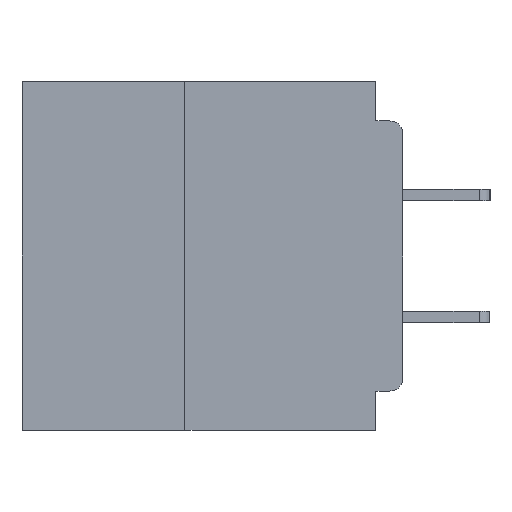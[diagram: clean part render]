
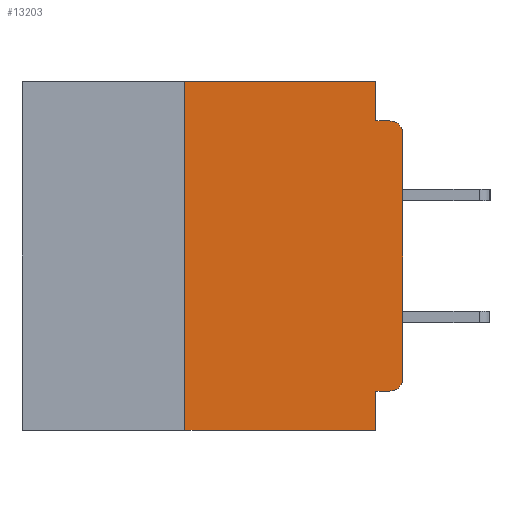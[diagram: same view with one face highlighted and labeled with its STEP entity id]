
A CAD part, left-side view. The second image highlights one B-rep face of the part: STEP entity #13203.
In plain terms, the highlighted planar face has unit normal (-1, 0, 0).
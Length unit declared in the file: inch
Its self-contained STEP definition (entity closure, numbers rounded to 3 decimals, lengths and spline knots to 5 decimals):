
#401 = VERTEX_POINT ( 'NONE', #18178 ) ;
#809 = ORIENTED_EDGE ( 'NONE', *, *, #40413, .F. ) ;
#1559 = EDGE_CURVE ( 'NONE', #32634, #18554, #17496, .T. ) ;
#2221 = CARTESIAN_POINT ( 'NONE',  ( 0., 0.25, 0. ) ) ;
#2320 = EDGE_CURVE ( 'NONE', #28831, #16118, #28950, .T. ) ;
#2930 = EDGE_CURVE ( 'NONE', #31306, #37913, #16008, .T. ) ;
#3316 = DIRECTION ( 'NONE',  ( 0., 1., 0. ) ) ;
#5007 = VECTOR ( 'NONE', #46471, 39.37008 ) ;
#5088 = ORIENTED_EDGE ( 'NONE', *, *, #42461, .F. ) ;
#6559 = CARTESIAN_POINT ( 'NONE',  ( 0., 0.015, -0.34 ) ) ;
#6659 = EDGE_LOOP ( 'NONE', ( #49998, #7656, #8970, #49435, #10941, #5088, #35610, #40774, #809, #45918 ) ) ;
#7120 = DIRECTION ( 'NONE',  ( 0., 0., -1. ) ) ;
#7656 = ORIENTED_EDGE ( 'NONE', *, *, #42361, .T. ) ;
#8857 = DIRECTION ( 'NONE',  ( -1., 0., 0. ) ) ;
#8970 = ORIENTED_EDGE ( 'NONE', *, *, #17327, .F. ) ;
#8975 = CARTESIAN_POINT ( 'NONE',  ( 0., 0.437, 0. ) ) ;
#9011 = LINE ( 'NONE', #48057, #50084 ) ;
#9158 = DIRECTION ( 'NONE',  ( 1., 0., 0. ) ) ;
#9798 = AXIS2_PLACEMENT_3D ( 'NONE', #8975, #9158, #37834 ) ;
#10071 = CARTESIAN_POINT ( 'NONE',  ( 0., 0., -0.045 ) ) ;
#10750 = DIRECTION ( 'NONE',  ( 0., 0., -1. ) ) ;
#10759 = VERTEX_POINT ( 'NONE', #27422 ) ;
#10941 = ORIENTED_EDGE ( 'NONE', *, *, #2930, .F. ) ;
#12229 = CARTESIAN_POINT ( 'NONE',  ( 0., 0.25, -0.4 ) ) ;
#13144 = PLANE ( 'NONE',  #9798 ) ;
#13203 = ADVANCED_FACE ( 'NONE', ( #36014 ), #13144, .F. ) ;
#13788 = CIRCLE ( 'NONE', #38934, 0.015 ) ;
#16008 = LINE ( 'NONE', #37794, #5007 ) ;
#16118 = VERTEX_POINT ( 'NONE', #30633 ) ;
#16352 = DIRECTION ( 'NONE',  ( 0., 0., 1. ) ) ;
#17327 = EDGE_CURVE ( 'NONE', #10759, #34724, #40458, .T. ) ;
#17496 = LINE ( 'NONE', #43447, #37992 ) ;
#18178 = CARTESIAN_POINT ( 'NONE',  ( 0., 0.031, -0.355 ) ) ;
#18554 = VERTEX_POINT ( 'NONE', #21112 ) ;
#21112 = CARTESIAN_POINT ( 'NONE',  ( 0., 0.031, -0.4 ) ) ;
#21429 = VECTOR ( 'NONE', #36794, 39.37008 ) ;
#23556 = CARTESIAN_POINT ( 'NONE',  ( 0., 0., -0.34 ) ) ;
#27181 = CARTESIAN_POINT ( 'NONE',  ( 0., 0.25, -0.4 ) ) ;
#27422 = CARTESIAN_POINT ( 'NONE',  ( 0., 0.031, -0.045 ) ) ;
#28530 = VERTEX_POINT ( 'NONE', #46315 ) ;
#28831 = VERTEX_POINT ( 'NONE', #23556 ) ;
#28871 = CARTESIAN_POINT ( 'NONE',  ( 0., 0., 0. ) ) ;
#28950 = LINE ( 'NONE', #28871, #48158 ) ;
#29394 = EDGE_CURVE ( 'NONE', #28530, #28831, #13788, .T. ) ;
#29843 = CIRCLE ( 'NONE', #41533, 0.015 ) ;
#30141 = CARTESIAN_POINT ( 'NONE',  ( 0., 0.015, -0.045 ) ) ;
#30633 = CARTESIAN_POINT ( 'NONE',  ( 0., 0., -0.06 ) ) ;
#31306 = VERTEX_POINT ( 'NONE', #2221 ) ;
#31428 = EDGE_CURVE ( 'NONE', #401, #18554, #9011, .T. ) ;
#32106 = CARTESIAN_POINT ( 'NONE',  ( 0., 0., -0.355 ) ) ;
#32385 = CARTESIAN_POINT ( 'NONE',  ( 0., 0.031, 0. ) ) ;
#32634 = VERTEX_POINT ( 'NONE', #27181 ) ;
#33170 = VECTOR ( 'NONE', #3316, 39.37008 ) ;
#33432 = CARTESIAN_POINT ( 'NONE',  ( 0., 0.015, -0.06 ) ) ;
#33989 = EDGE_CURVE ( 'NONE', #37913, #10759, #39361, .T. ) ;
#34598 = DIRECTION ( 'NONE',  ( 0., -1., 0. ) ) ;
#34724 = VERTEX_POINT ( 'NONE', #30141 ) ;
#35280 = DIRECTION ( 'NONE',  ( -1., 0., 0. ) ) ;
#35610 = ORIENTED_EDGE ( 'NONE', *, *, #1559, .T. ) ;
#36014 = FACE_OUTER_BOUND ( 'NONE', #6659, .T. ) ;
#36794 = DIRECTION ( 'NONE',  ( 0., 0., -1. ) ) ;
#37555 = DIRECTION ( 'NONE',  ( 0., 0., -1. ) ) ;
#37794 = CARTESIAN_POINT ( 'NONE',  ( 0., 0.437, 0. ) ) ;
#37834 = DIRECTION ( 'NONE',  ( 0., 0., -1. ) ) ;
#37913 = VERTEX_POINT ( 'NONE', #32385 ) ;
#37992 = VECTOR ( 'NONE', #46339, 39.37008 ) ;
#38934 = AXIS2_PLACEMENT_3D ( 'NONE', #6559, #35280, #10750 ) ;
#39361 = LINE ( 'NONE', #49193, #21429 ) ;
#40413 = EDGE_CURVE ( 'NONE', #28530, #401, #45353, .T. ) ;
#40458 = LINE ( 'NONE', #10071, #50102 ) ;
#40774 = ORIENTED_EDGE ( 'NONE', *, *, #31428, .F. ) ;
#41533 = AXIS2_PLACEMENT_3D ( 'NONE', #33432, #8857, #37555 ) ;
#42361 = EDGE_CURVE ( 'NONE', #16118, #34724, #29843, .T. ) ;
#42461 = EDGE_CURVE ( 'NONE', #32634, #31306, #43189, .T. ) ;
#43189 = LINE ( 'NONE', #12229, #52841 ) ;
#43447 = CARTESIAN_POINT ( 'NONE',  ( 0., 0.437, -0.4 ) ) ;
#45353 = LINE ( 'NONE', #32106, #33170 ) ;
#45918 = ORIENTED_EDGE ( 'NONE', *, *, #29394, .T. ) ;
#46315 = CARTESIAN_POINT ( 'NONE',  ( 0., 0.015, -0.355 ) ) ;
#46339 = DIRECTION ( 'NONE',  ( 0., -1., 0. ) ) ;
#46471 = DIRECTION ( 'NONE',  ( 0., -1., 0. ) ) ;
#48057 = CARTESIAN_POINT ( 'NONE',  ( 0., 0.031, -0.4 ) ) ;
#48158 = VECTOR ( 'NONE', #48442, 39.37008 ) ;
#48442 = DIRECTION ( 'NONE',  ( 0., 0., 1. ) ) ;
#49193 = CARTESIAN_POINT ( 'NONE',  ( 0., 0.031, 0. ) ) ;
#49435 = ORIENTED_EDGE ( 'NONE', *, *, #33989, .F. ) ;
#49998 = ORIENTED_EDGE ( 'NONE', *, *, #2320, .T. ) ;
#50084 = VECTOR ( 'NONE', #7120, 39.37008 ) ;
#50102 = VECTOR ( 'NONE', #34598, 39.37008 ) ;
#52841 = VECTOR ( 'NONE', #16352, 39.37008 ) ;
